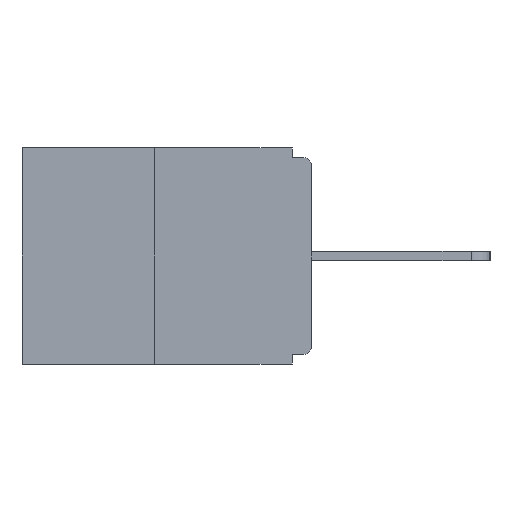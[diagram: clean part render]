
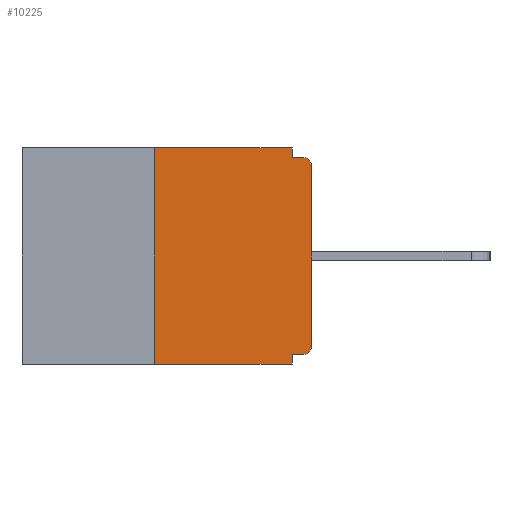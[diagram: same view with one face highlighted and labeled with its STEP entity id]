
A CAD part, left-side view. The second image highlights one B-rep face of the part: STEP entity #10225.
In plain terms, the highlighted planar face has unit normal (-1, 0, 0).
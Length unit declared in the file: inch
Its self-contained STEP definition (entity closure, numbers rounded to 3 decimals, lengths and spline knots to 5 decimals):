
#49 = CARTESIAN_POINT ( 'NONE',  ( 0., 0., -0.313 ) ) ;
#56 = ORIENTED_EDGE ( 'NONE', *, *, #613, .F. ) ;
#174 = CARTESIAN_POINT ( 'NONE',  ( 0., 0.015, -0.328 ) ) ;
#404 = CARTESIAN_POINT ( 'NONE',  ( 0., 0.46, 0. ) ) ;
#613 = EDGE_CURVE ( 'NONE', #2781, #24592, #20393, .T. ) ;
#848 = CARTESIAN_POINT ( 'NONE',  ( 0., 0., -0.03 ) ) ;
#1176 = LINE ( 'NONE', #12225, #21311 ) ;
#1193 = EDGE_CURVE ( 'NONE', #10605, #9851, #20984, .T. ) ;
#1542 = VERTEX_POINT ( 'NONE', #12460 ) ;
#2086 = CARTESIAN_POINT ( 'NONE',  ( 0., 0.031, 0. ) ) ;
#2113 = EDGE_CURVE ( 'NONE', #1542, #21363, #24929, .T. ) ;
#2367 = CARTESIAN_POINT ( 'NONE',  ( 0., 0.25, 0. ) ) ;
#2399 = CARTESIAN_POINT ( 'NONE',  ( 0., 0.031, 0. ) ) ;
#2407 = EDGE_CURVE ( 'NONE', #10653, #20378, #16316, .T. ) ;
#2781 = VERTEX_POINT ( 'NONE', #6255 ) ;
#3398 = CARTESIAN_POINT ( 'NONE',  ( 0., 0.46, 0. ) ) ;
#4106 = CARTESIAN_POINT ( 'NONE',  ( 0., 0.031, -0.343 ) ) ;
#4312 = AXIS2_PLACEMENT_3D ( 'NONE', #23528, #9794, #17917 ) ;
#4314 = EDGE_CURVE ( 'NONE', #20378, #17851, #6136, .T. ) ;
#5258 = ORIENTED_EDGE ( 'NONE', *, *, #6249, .T. ) ;
#5449 = DIRECTION ( 'NONE',  ( 0., 0., -1. ) ) ;
#5472 = EDGE_CURVE ( 'NONE', #10653, #2781, #22124, .T. ) ;
#5536 = DIRECTION ( 'NONE',  ( 1., 0., 0. ) ) ;
#5795 = AXIS2_PLACEMENT_3D ( 'NONE', #18188, #14310, #12682 ) ;
#6107 = ORIENTED_EDGE ( 'NONE', *, *, #9664, .F. ) ;
#6136 = LINE ( 'NONE', #8788, #22610 ) ;
#6249 = EDGE_CURVE ( 'NONE', #1542, #24592, #1176, .T. ) ;
#6255 = CARTESIAN_POINT ( 'NONE',  ( 0., 0.031, -0.328 ) ) ;
#6256 = VECTOR ( 'NONE', #6874, 39.37008 ) ;
#6580 = DIRECTION ( 'NONE',  ( 0., -1., 0. ) ) ;
#6840 = LINE ( 'NONE', #2086, #6256 ) ;
#6874 = DIRECTION ( 'NONE',  ( 0., 0., -1. ) ) ;
#7675 = DIRECTION ( 'NONE',  ( 0., 0., 1. ) ) ;
#8788 = CARTESIAN_POINT ( 'NONE',  ( 0., 0., 0. ) ) ;
#9620 = CIRCLE ( 'NONE', #4312, 0.015 ) ;
#9664 = EDGE_CURVE ( 'NONE', #23470, #10605, #6840, .T. ) ;
#9794 = DIRECTION ( 'NONE',  ( -1., 0., 0. ) ) ;
#9851 = VERTEX_POINT ( 'NONE', #18312 ) ;
#9953 = DIRECTION ( 'NONE',  ( 0., -1., 0. ) ) ;
#10091 = EDGE_CURVE ( 'NONE', #21363, #23470, #23982, .T. ) ;
#10225 = ADVANCED_FACE ( 'NONE', ( #12068 ), #18980, .F. ) ;
#10605 = VERTEX_POINT ( 'NONE', #21301 ) ;
#10653 = VERTEX_POINT ( 'NONE', #174 ) ;
#11717 = CARTESIAN_POINT ( 'NONE',  ( 0., 0.25, 0. ) ) ;
#11869 = CARTESIAN_POINT ( 'NONE',  ( 0., 0., -0.328 ) ) ;
#12068 = FACE_OUTER_BOUND ( 'NONE', #22818, .T. ) ;
#12225 = CARTESIAN_POINT ( 'NONE',  ( 0., 0.46, -0.343 ) ) ;
#12460 = CARTESIAN_POINT ( 'NONE',  ( 0., 0.25, -0.343 ) ) ;
#12682 = DIRECTION ( 'NONE',  ( 0., 0., -1. ) ) ;
#12973 = VECTOR ( 'NONE', #9953, 39.37008 ) ;
#13946 = VECTOR ( 'NONE', #7675, 39.37008 ) ;
#14124 = EDGE_CURVE ( 'NONE', #17851, #9851, #9620, .T. ) ;
#14310 = DIRECTION ( 'NONE',  ( -1., 0., 0. ) ) ;
#14360 = CARTESIAN_POINT ( 'NONE',  ( 0., 0., -0.015 ) ) ;
#15686 = ORIENTED_EDGE ( 'NONE', *, *, #2407, .T. ) ;
#16292 = DIRECTION ( 'NONE',  ( 0., -1., 0. ) ) ;
#16316 = CIRCLE ( 'NONE', #5795, 0.015 ) ;
#17851 = VERTEX_POINT ( 'NONE', #848 ) ;
#17917 = DIRECTION ( 'NONE',  ( 0., 0., -1. ) ) ;
#17926 = VECTOR ( 'NONE', #5449, 39.37008 ) ;
#18188 = CARTESIAN_POINT ( 'NONE',  ( 0., 0.015, -0.313 ) ) ;
#18312 = CARTESIAN_POINT ( 'NONE',  ( 0., 0.015, -0.015 ) ) ;
#18980 = PLANE ( 'NONE',  #19240 ) ;
#19034 = VECTOR ( 'NONE', #21899, 39.37008 ) ;
#19155 = DIRECTION ( 'NONE',  ( 0., 0., -1. ) ) ;
#19240 = AXIS2_PLACEMENT_3D ( 'NONE', #3398, #5536, #19155 ) ;
#19371 = ORIENTED_EDGE ( 'NONE', *, *, #10091, .F. ) ;
#20367 = ORIENTED_EDGE ( 'NONE', *, *, #2113, .F. ) ;
#20372 = VECTOR ( 'NONE', #6580, 39.37008 ) ;
#20378 = VERTEX_POINT ( 'NONE', #49 ) ;
#20391 = ORIENTED_EDGE ( 'NONE', *, *, #4314, .T. ) ;
#20393 = LINE ( 'NONE', #4106, #17926 ) ;
#20457 = CARTESIAN_POINT ( 'NONE',  ( 0., 0.031, -0.343 ) ) ;
#20524 = DIRECTION ( 'NONE',  ( 0., 0., 1. ) ) ;
#20984 = LINE ( 'NONE', #14360, #20372 ) ;
#21301 = CARTESIAN_POINT ( 'NONE',  ( 0., 0.031, -0.015 ) ) ;
#21311 = VECTOR ( 'NONE', #16292, 39.37008 ) ;
#21363 = VERTEX_POINT ( 'NONE', #2367 ) ;
#21899 = DIRECTION ( 'NONE',  ( 0., 1., 0. ) ) ;
#22124 = LINE ( 'NONE', #11869, #19034 ) ;
#22171 = ORIENTED_EDGE ( 'NONE', *, *, #1193, .F. ) ;
#22610 = VECTOR ( 'NONE', #20524, 39.37008 ) ;
#22818 = EDGE_LOOP ( 'NONE', ( #19371, #20367, #5258, #56, #25039, #15686, #20391, #23150, #22171, #6107 ) ) ;
#23150 = ORIENTED_EDGE ( 'NONE', *, *, #14124, .T. ) ;
#23470 = VERTEX_POINT ( 'NONE', #2399 ) ;
#23528 = CARTESIAN_POINT ( 'NONE',  ( 0., 0.015, -0.03 ) ) ;
#23982 = LINE ( 'NONE', #404, #12973 ) ;
#24592 = VERTEX_POINT ( 'NONE', #20457 ) ;
#24929 = LINE ( 'NONE', #11717, #13946 ) ;
#25039 = ORIENTED_EDGE ( 'NONE', *, *, #5472, .F. ) ;
